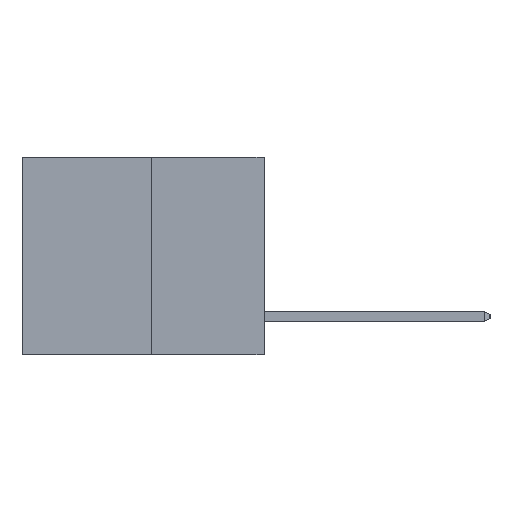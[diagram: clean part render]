
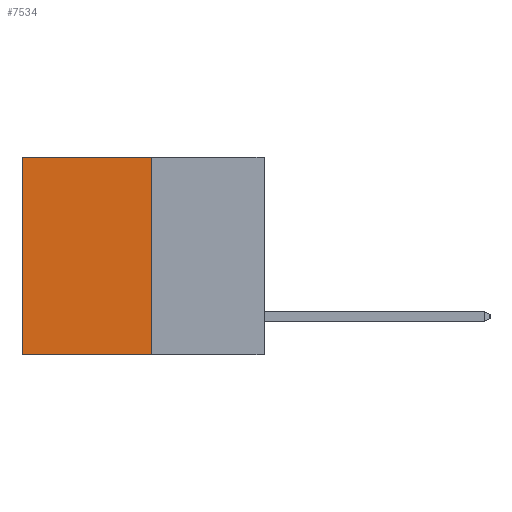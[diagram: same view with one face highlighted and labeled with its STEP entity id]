
A CAD part, left-side view. The second image highlights one B-rep face of the part: STEP entity #7534.
In plain terms, the highlighted planar face has unit normal (-1, 0, 0).
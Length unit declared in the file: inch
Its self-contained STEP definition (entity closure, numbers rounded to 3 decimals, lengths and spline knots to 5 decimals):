
#202 = EDGE_LOOP ( 'NONE', ( #12655, #16003, #3536, #14166 ) ) ;
#2578 = CARTESIAN_POINT ( 'NONE',  ( 0.3165, 0.28, -0.49 ) ) ;
#2839 = PLANE ( 'NONE',  #5816 ) ;
#3114 = VECTOR ( 'NONE', #20297, 39.37008 ) ;
#3536 = ORIENTED_EDGE ( 'NONE', *, *, #19955, .F. ) ;
#4494 = VECTOR ( 'NONE', #16062, 39.37008 ) ;
#4541 = DIRECTION ( 'NONE',  ( 0., 0., -1. ) ) ;
#4543 = CARTESIAN_POINT ( 'NONE',  ( 0.3165, 0.28, -0.49 ) ) ;
#5752 = CARTESIAN_POINT ( 'NONE',  ( 0.3165, 0.6, -0.49 ) ) ;
#5816 = AXIS2_PLACEMENT_3D ( 'NONE', #18364, #11440, #4541 ) ;
#5913 = CARTESIAN_POINT ( 'NONE',  ( 0.3165, 0.6, -0.49 ) ) ;
#7534 = ADVANCED_FACE ( 'NONE', ( #12606 ), #2839, .F. ) ;
#8406 = EDGE_CURVE ( 'NONE', #17893, #11217, #22290, .T. ) ;
#9743 = LINE ( 'NONE', #4543, #21069 ) ;
#9759 = EDGE_CURVE ( 'NONE', #11217, #17253, #18188, .T. ) ;
#10081 = VERTEX_POINT ( 'NONE', #21194 ) ;
#11217 = VERTEX_POINT ( 'NONE', #19924 ) ;
#11440 = DIRECTION ( 'NONE',  ( 1., 0., 0. ) ) ;
#11880 = CARTESIAN_POINT ( 'NONE',  ( 0.3165, 0.28, 0. ) ) ;
#12594 = LINE ( 'NONE', #2578, #4494 ) ;
#12606 = FACE_OUTER_BOUND ( 'NONE', #202, .T. ) ;
#12655 = ORIENTED_EDGE ( 'NONE', *, *, #9759, .T. ) ;
#14166 = ORIENTED_EDGE ( 'NONE', *, *, #8406, .T. ) ;
#14510 = EDGE_CURVE ( 'NONE', #10081, #17253, #12594, .T. ) ;
#14665 = DIRECTION ( 'NONE',  ( 0., 0., -1. ) ) ;
#15477 = CARTESIAN_POINT ( 'NONE',  ( 0.3165, 0.28, 0. ) ) ;
#15751 = VECTOR ( 'NONE', #14665, 39.37008 ) ;
#16003 = ORIENTED_EDGE ( 'NONE', *, *, #14510, .F. ) ;
#16062 = DIRECTION ( 'NONE',  ( 0., 1., 0. ) ) ;
#16334 = DIRECTION ( 'NONE',  ( 0., 0., -1. ) ) ;
#17253 = VERTEX_POINT ( 'NONE', #5752 ) ;
#17893 = VERTEX_POINT ( 'NONE', #11880 ) ;
#18188 = LINE ( 'NONE', #5913, #15751 ) ;
#18364 = CARTESIAN_POINT ( 'NONE',  ( 0.3165, 0.28, -0.49 ) ) ;
#19924 = CARTESIAN_POINT ( 'NONE',  ( 0.3165, 0.6, 0. ) ) ;
#19955 = EDGE_CURVE ( 'NONE', #17893, #10081, #9743, .T. ) ;
#20297 = DIRECTION ( 'NONE',  ( 0., 1., 0. ) ) ;
#21069 = VECTOR ( 'NONE', #16334, 39.37008 ) ;
#21194 = CARTESIAN_POINT ( 'NONE',  ( 0.3165, 0.28, -0.49 ) ) ;
#22290 = LINE ( 'NONE', #15477, #3114 ) ;
